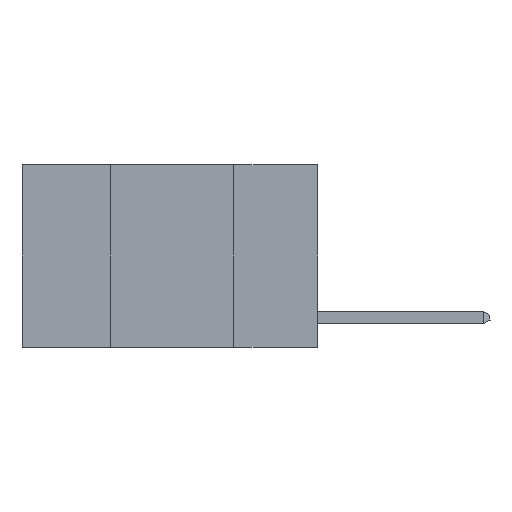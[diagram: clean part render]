
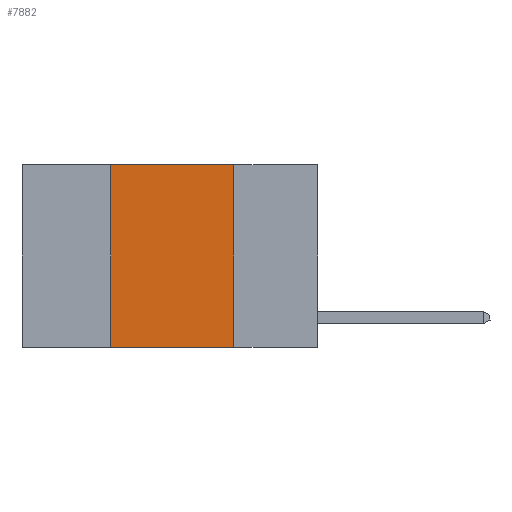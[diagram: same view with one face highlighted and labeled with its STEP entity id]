
A CAD part, left-side view. The second image highlights one B-rep face of the part: STEP entity #7882.
In plain terms, the highlighted planar face has unit normal (-1, 0, 0).
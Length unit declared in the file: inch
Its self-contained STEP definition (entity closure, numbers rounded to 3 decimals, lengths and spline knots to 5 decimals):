
#405 = VECTOR ( 'NONE', #1177, 39.37008 ) ;
#736 = FACE_OUTER_BOUND ( 'NONE', #3417, .T. ) ;
#770 = DIRECTION ( 'NONE',  ( 0., -1., 0. ) ) ;
#1177 = DIRECTION ( 'NONE',  ( 0., -1., 0. ) ) ;
#1216 = CARTESIAN_POINT ( 'NONE',  ( 0., 0.42, 0. ) ) ;
#2345 = CARTESIAN_POINT ( 'NONE',  ( 0., 0.42, -0.37 ) ) ;
#2756 = LINE ( 'NONE', #3783, #405 ) ;
#3100 = DIRECTION ( 'NONE',  ( 0., 0., 1. ) ) ;
#3234 = VERTEX_POINT ( 'NONE', #4540 ) ;
#3241 = VECTOR ( 'NONE', #10739, 39.37008 ) ;
#3417 = EDGE_LOOP ( 'NONE', ( #4403, #6653, #10826, #4686 ) ) ;
#3447 = DIRECTION ( 'NONE',  ( 1., 0., 0. ) ) ;
#3783 = CARTESIAN_POINT ( 'NONE',  ( 0., 0.6, -0.37 ) ) ;
#4082 = VERTEX_POINT ( 'NONE', #2345 ) ;
#4165 = VECTOR ( 'NONE', #770, 39.37008 ) ;
#4268 = CARTESIAN_POINT ( 'NONE',  ( 0., 0.17, 0. ) ) ;
#4403 = ORIENTED_EDGE ( 'NONE', *, *, #7223, .F. ) ;
#4540 = CARTESIAN_POINT ( 'NONE',  ( 0., 0.17, -0.37 ) ) ;
#4686 = ORIENTED_EDGE ( 'NONE', *, *, #8847, .T. ) ;
#5208 = CARTESIAN_POINT ( 'NONE',  ( 0., 0.6, 0. ) ) ;
#6061 = VERTEX_POINT ( 'NONE', #1216 ) ;
#6653 = ORIENTED_EDGE ( 'NONE', *, *, #10728, .F. ) ;
#6692 = LINE ( 'NONE', #5208, #4165 ) ;
#6982 = VERTEX_POINT ( 'NONE', #10451 ) ;
#7051 = EDGE_CURVE ( 'NONE', #4082, #6061, #9007, .T. ) ;
#7142 = VECTOR ( 'NONE', #3100, 39.37008 ) ;
#7223 = EDGE_CURVE ( 'NONE', #6982, #3234, #8012, .T. ) ;
#7611 = CARTESIAN_POINT ( 'NONE',  ( 0., 0.6, 0. ) ) ;
#7673 = PLANE ( 'NONE',  #8703 ) ;
#7882 = ADVANCED_FACE ( 'NONE', ( #736 ), #7673, .F. ) ;
#8012 = LINE ( 'NONE', #4268, #3241 ) ;
#8215 = CARTESIAN_POINT ( 'NONE',  ( 0., 0.42, 0. ) ) ;
#8703 = AXIS2_PLACEMENT_3D ( 'NONE', #7611, #3447, #9271 ) ;
#8847 = EDGE_CURVE ( 'NONE', #4082, #3234, #2756, .T. ) ;
#9007 = LINE ( 'NONE', #8215, #7142 ) ;
#9271 = DIRECTION ( 'NONE',  ( 0., 0., -1. ) ) ;
#10451 = CARTESIAN_POINT ( 'NONE',  ( 0., 0.17, 0. ) ) ;
#10728 = EDGE_CURVE ( 'NONE', #6061, #6982, #6692, .T. ) ;
#10739 = DIRECTION ( 'NONE',  ( 0., 0., -1. ) ) ;
#10826 = ORIENTED_EDGE ( 'NONE', *, *, #7051, .F. ) ;
